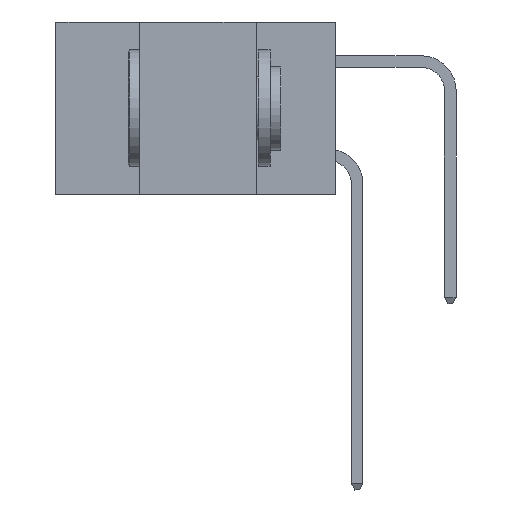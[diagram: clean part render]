
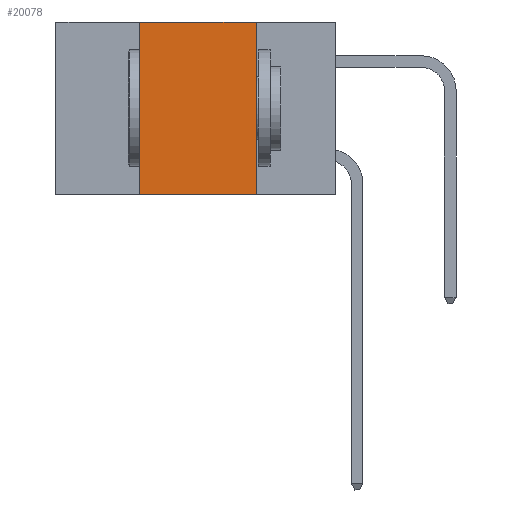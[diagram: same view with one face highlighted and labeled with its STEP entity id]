
A CAD part, left-side view. The second image highlights one B-rep face of the part: STEP entity #20078.
In plain terms, the highlighted planar face has unit normal (-1, 0, 0).
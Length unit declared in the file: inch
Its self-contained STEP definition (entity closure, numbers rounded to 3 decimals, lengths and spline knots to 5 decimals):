
#984 = VECTOR ( 'NONE', #25071, 39.37008 ) ;
#2181 = DIRECTION ( 'NONE',  ( 0., 0., -1. ) ) ;
#2780 = VECTOR ( 'NONE', #18733, 39.37008 ) ;
#5312 = CARTESIAN_POINT ( 'NONE',  ( 0., 0.6, -0.37 ) ) ;
#5394 = ORIENTED_EDGE ( 'NONE', *, *, #23731, .F. ) ;
#5829 = DIRECTION ( 'NONE',  ( 0., 0., -1. ) ) ;
#6087 = VERTEX_POINT ( 'NONE', #9153 ) ;
#6259 = LINE ( 'NONE', #24856, #2780 ) ;
#7270 = ORIENTED_EDGE ( 'NONE', *, *, #21202, .T. ) ;
#7896 = VECTOR ( 'NONE', #2181, 39.37008 ) ;
#8502 = EDGE_CURVE ( 'NONE', #18009, #6087, #6259, .T. ) ;
#8581 = CARTESIAN_POINT ( 'NONE',  ( 0., 0.42, 0. ) ) ;
#9153 = CARTESIAN_POINT ( 'NONE',  ( 0., 0.17, 0. ) ) ;
#9844 = PLANE ( 'NONE',  #11082 ) ;
#10585 = VERTEX_POINT ( 'NONE', #19127 ) ;
#11082 = AXIS2_PLACEMENT_3D ( 'NONE', #26029, #15911, #5829 ) ;
#11125 = EDGE_LOOP ( 'NONE', ( #19343, #15862, #5394, #7270 ) ) ;
#14478 = LINE ( 'NONE', #5312, #24639 ) ;
#15862 = ORIENTED_EDGE ( 'NONE', *, *, #8502, .F. ) ;
#15911 = DIRECTION ( 'NONE',  ( 1., 0., 0. ) ) ;
#17553 = EDGE_CURVE ( 'NONE', #6087, #26144, #24114, .T. ) ;
#18009 = VERTEX_POINT ( 'NONE', #19744 ) ;
#18733 = DIRECTION ( 'NONE',  ( 0., -1., 0. ) ) ;
#19127 = CARTESIAN_POINT ( 'NONE',  ( 0., 0.42, -0.37 ) ) ;
#19343 = ORIENTED_EDGE ( 'NONE', *, *, #17553, .F. ) ;
#19744 = CARTESIAN_POINT ( 'NONE',  ( 0., 0.42, 0. ) ) ;
#20078 = ADVANCED_FACE ( 'NONE', ( #23014 ), #9844, .F. ) ;
#20223 = CARTESIAN_POINT ( 'NONE',  ( 0., 0.17, 0. ) ) ;
#21202 = EDGE_CURVE ( 'NONE', #10585, #26144, #14478, .T. ) ;
#23014 = FACE_OUTER_BOUND ( 'NONE', #11125, .T. ) ;
#23603 = DIRECTION ( 'NONE',  ( 0., -1., 0. ) ) ;
#23731 = EDGE_CURVE ( 'NONE', #10585, #18009, #24515, .T. ) ;
#24114 = LINE ( 'NONE', #20223, #7896 ) ;
#24131 = CARTESIAN_POINT ( 'NONE',  ( 0., 0.17, -0.37 ) ) ;
#24515 = LINE ( 'NONE', #8581, #984 ) ;
#24639 = VECTOR ( 'NONE', #23603, 39.37008 ) ;
#24856 = CARTESIAN_POINT ( 'NONE',  ( 0., 0.6, 0. ) ) ;
#25071 = DIRECTION ( 'NONE',  ( 0., 0., 1. ) ) ;
#26029 = CARTESIAN_POINT ( 'NONE',  ( 0., 0.6, 0. ) ) ;
#26144 = VERTEX_POINT ( 'NONE', #24131 ) ;
